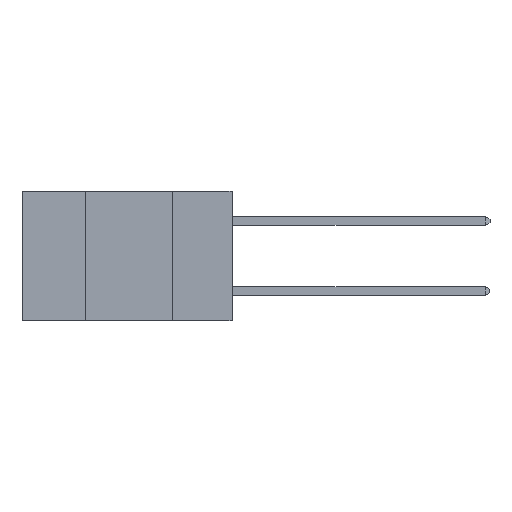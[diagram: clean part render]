
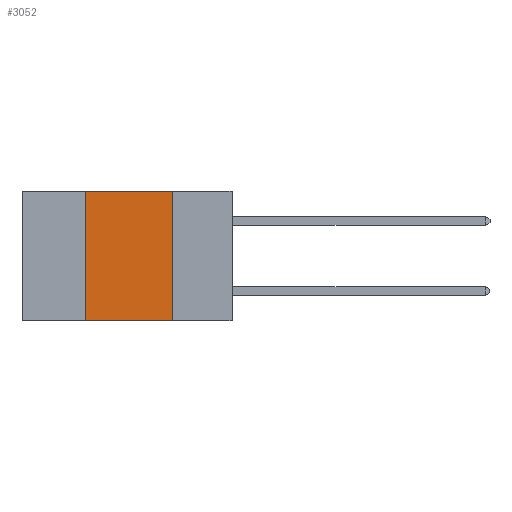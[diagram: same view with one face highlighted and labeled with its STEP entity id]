
A CAD part, left-side view. The second image highlights one B-rep face of the part: STEP entity #3052.
In plain terms, the highlighted planar face has unit normal (-1, 0, 0).
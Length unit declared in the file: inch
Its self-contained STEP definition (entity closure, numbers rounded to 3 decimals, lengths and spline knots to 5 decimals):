
#37 = VERTEX_POINT ( 'NONE', #8252 ) ;
#406 = CARTESIAN_POINT ( 'NONE',  ( 0., 0.42, 0. ) ) ;
#642 = ORIENTED_EDGE ( 'NONE', *, *, #5025, .F. ) ;
#1266 = DIRECTION ( 'NONE',  ( 1., 0., 0. ) ) ;
#1608 = CARTESIAN_POINT ( 'NONE',  ( 0., 0.6, 0. ) ) ;
#1783 = VECTOR ( 'NONE', #11982, 39.37008 ) ;
#2540 = VECTOR ( 'NONE', #7137, 39.37008 ) ;
#3052 = ADVANCED_FACE ( 'NONE', ( #9580 ), #6811, .F. ) ;
#3200 = ORIENTED_EDGE ( 'NONE', *, *, #6419, .F. ) ;
#3263 = VERTEX_POINT ( 'NONE', #10743 ) ;
#3766 = VECTOR ( 'NONE', #6038, 39.37008 ) ;
#4093 = ORIENTED_EDGE ( 'NONE', *, *, #5154, .F. ) ;
#4726 = VERTEX_POINT ( 'NONE', #5641 ) ;
#4904 = CARTESIAN_POINT ( 'NONE',  ( 0., 0.42, -0.37 ) ) ;
#5025 = EDGE_CURVE ( 'NONE', #9885, #4726, #6979, .T. ) ;
#5154 = EDGE_CURVE ( 'NONE', #4726, #3263, #9199, .T. ) ;
#5389 = EDGE_CURVE ( 'NONE', #9885, #37, #11814, .T. ) ;
#5641 = CARTESIAN_POINT ( 'NONE',  ( 0., 0.42, 0. ) ) ;
#5659 = EDGE_LOOP ( 'NONE', ( #3200, #4093, #642, #11034 ) ) ;
#5802 = AXIS2_PLACEMENT_3D ( 'NONE', #5882, #1266, #7737 ) ;
#5882 = CARTESIAN_POINT ( 'NONE',  ( 0., 0.6, 0. ) ) ;
#6038 = DIRECTION ( 'NONE',  ( 0., 0., 1. ) ) ;
#6419 = EDGE_CURVE ( 'NONE', #3263, #37, #9780, .T. ) ;
#6811 = PLANE ( 'NONE',  #5802 ) ;
#6979 = LINE ( 'NONE', #406, #3766 ) ;
#7137 = DIRECTION ( 'NONE',  ( 0., -1., 0. ) ) ;
#7363 = VECTOR ( 'NONE', #9394, 39.37008 ) ;
#7737 = DIRECTION ( 'NONE',  ( 0., 0., -1. ) ) ;
#8252 = CARTESIAN_POINT ( 'NONE',  ( 0., 0.17, -0.37 ) ) ;
#9189 = CARTESIAN_POINT ( 'NONE',  ( 0., 0.6, -0.37 ) ) ;
#9199 = LINE ( 'NONE', #1608, #2540 ) ;
#9394 = DIRECTION ( 'NONE',  ( 0., 0., -1. ) ) ;
#9580 = FACE_OUTER_BOUND ( 'NONE', #5659, .T. ) ;
#9780 = LINE ( 'NONE', #11213, #7363 ) ;
#9885 = VERTEX_POINT ( 'NONE', #4904 ) ;
#10743 = CARTESIAN_POINT ( 'NONE',  ( 0., 0.17, 0. ) ) ;
#11034 = ORIENTED_EDGE ( 'NONE', *, *, #5389, .T. ) ;
#11213 = CARTESIAN_POINT ( 'NONE',  ( 0., 0.17, 0. ) ) ;
#11814 = LINE ( 'NONE', #9189, #1783 ) ;
#11982 = DIRECTION ( 'NONE',  ( 0., -1., 0. ) ) ;
